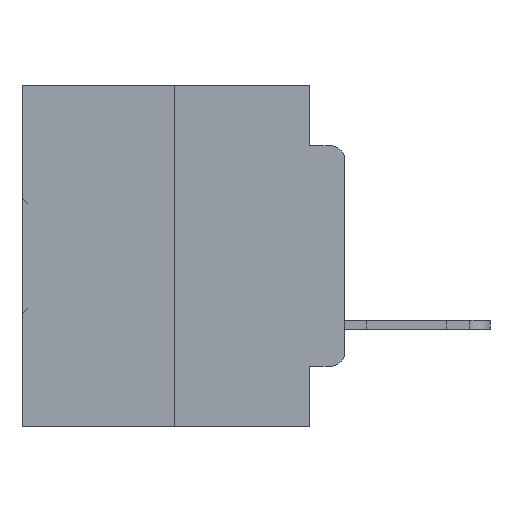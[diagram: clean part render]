
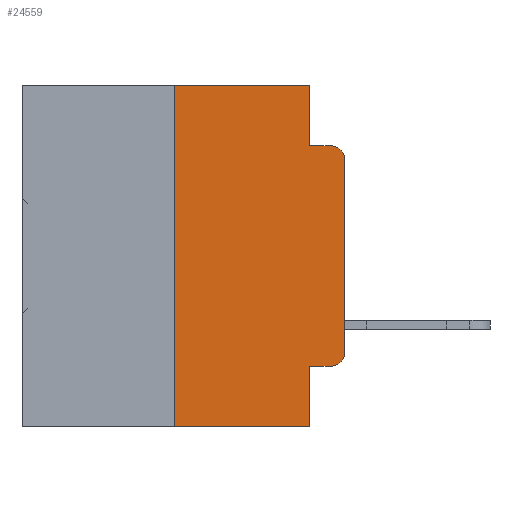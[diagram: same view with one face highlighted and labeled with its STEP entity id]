
A CAD part, left-side view. The second image highlights one B-rep face of the part: STEP entity #24559.
In plain terms, the highlighted planar face has unit normal (-1, 0, 0).
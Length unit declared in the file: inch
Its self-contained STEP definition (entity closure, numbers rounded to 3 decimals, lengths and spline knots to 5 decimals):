
#37 = VECTOR ( 'NONE', #6086, 39.37008 ) ;
#75 = CARTESIAN_POINT ( 'NONE',  ( 0., 0., -0.1085 ) ) ;
#310 = VERTEX_POINT ( 'NONE', #8747 ) ;
#1279 = EDGE_CURVE ( 'NONE', #30486, #15452, #26075, .T. ) ;
#1689 = VECTOR ( 'NONE', #25598, 39.37008 ) ;
#1767 = AXIS2_PLACEMENT_3D ( 'NONE', #25927, #13124, #30879 ) ;
#1870 = CARTESIAN_POINT ( 'NONE',  ( 0., 0.051, 0. ) ) ;
#2720 = LINE ( 'NONE', #21372, #24766 ) ;
#3675 = CARTESIAN_POINT ( 'NONE',  ( 0., 0.051, -0.0885 ) ) ;
#3795 = EDGE_LOOP ( 'NONE', ( #9376, #19537, #5300, #15542, #13757, #17718, #26564, #5742, #23280, #32112 ) ) ;
#3878 = AXIS2_PLACEMENT_3D ( 'NONE', #20931, #21285, #21146 ) ;
#4592 = VECTOR ( 'NONE', #22595, 39.37008 ) ;
#4764 = DIRECTION ( 'NONE',  ( 0., -1., 0. ) ) ;
#4811 = EDGE_CURVE ( 'NONE', #8818, #32693, #23656, .T. ) ;
#5300 = ORIENTED_EDGE ( 'NONE', *, *, #24972, .F. ) ;
#5493 = LINE ( 'NONE', #21628, #31832 ) ;
#5742 = ORIENTED_EDGE ( 'NONE', *, *, #12688, .F. ) ;
#6024 = CARTESIAN_POINT ( 'NONE',  ( 0., 0.051, -0.0885 ) ) ;
#6086 = DIRECTION ( 'NONE',  ( 0., 0., 1. ) ) ;
#6209 = VERTEX_POINT ( 'NONE', #6024 ) ;
#6871 = EDGE_CURVE ( 'NONE', #13027, #8818, #5493, .T. ) ;
#7002 = FACE_OUTER_BOUND ( 'NONE', #3795, .T. ) ;
#7730 = CIRCLE ( 'NONE', #23079, 0.02 ) ;
#8050 = CARTESIAN_POINT ( 'NONE',  ( 0., 0., -0.3915 ) ) ;
#8088 = DIRECTION ( 'NONE',  ( -1., 0., 0. ) ) ;
#8747 = CARTESIAN_POINT ( 'NONE',  ( 0., 0.02, -0.0885 ) ) ;
#8818 = VERTEX_POINT ( 'NONE', #32492 ) ;
#9070 = LINE ( 'NONE', #17429, #23403 ) ;
#9376 = ORIENTED_EDGE ( 'NONE', *, *, #32946, .T. ) ;
#10203 = PLANE ( 'NONE',  #1767 ) ;
#12688 = EDGE_CURVE ( 'NONE', #13027, #26458, #23816, .T. ) ;
#13027 = VERTEX_POINT ( 'NONE', #31003 ) ;
#13124 = DIRECTION ( 'NONE',  ( 1., 0., 0. ) ) ;
#13318 = DIRECTION ( 'NONE',  ( 0., 0., -1. ) ) ;
#13400 = CARTESIAN_POINT ( 'NONE',  ( 0., 0.051, 0. ) ) ;
#13757 = ORIENTED_EDGE ( 'NONE', *, *, #1279, .F. ) ;
#14579 = EDGE_CURVE ( 'NONE', #19467, #30486, #9070, .T. ) ;
#15423 = CARTESIAN_POINT ( 'NONE',  ( 0., 0.25, 0. ) ) ;
#15434 = DIRECTION ( 'NONE',  ( 0., 0., 1. ) ) ;
#15452 = VERTEX_POINT ( 'NONE', #1870 ) ;
#15542 = ORIENTED_EDGE ( 'NONE', *, *, #18186, .F. ) ;
#17429 = CARTESIAN_POINT ( 'NONE',  ( 0., 0.25, 0. ) ) ;
#17718 = ORIENTED_EDGE ( 'NONE', *, *, #14579, .F. ) ;
#17980 = EDGE_CURVE ( 'NONE', #19467, #26458, #2720, .T. ) ;
#18186 = EDGE_CURVE ( 'NONE', #15452, #6209, #25530, .T. ) ;
#19467 = VERTEX_POINT ( 'NONE', #27934 ) ;
#19537 = ORIENTED_EDGE ( 'NONE', *, *, #26612, .T. ) ;
#20770 = DIRECTION ( 'NONE',  ( 0., -1., 0. ) ) ;
#20931 = CARTESIAN_POINT ( 'NONE',  ( 0., 0.02, -0.3915 ) ) ;
#21146 = DIRECTION ( 'NONE',  ( 0., 0., -1. ) ) ;
#21285 = DIRECTION ( 'NONE',  ( -1., 0., 0. ) ) ;
#21372 = CARTESIAN_POINT ( 'NONE',  ( 0., 0.473, -0.5 ) ) ;
#21628 = CARTESIAN_POINT ( 'NONE',  ( 0., 0.051, -0.4115 ) ) ;
#22435 = LINE ( 'NONE', #29793, #37 ) ;
#22595 = DIRECTION ( 'NONE',  ( 0., 0., -1. ) ) ;
#22991 = VECTOR ( 'NONE', #13318, 39.37008 ) ;
#23079 = AXIS2_PLACEMENT_3D ( 'NONE', #24226, #8088, #26688 ) ;
#23280 = ORIENTED_EDGE ( 'NONE', *, *, #6871, .T. ) ;
#23403 = VECTOR ( 'NONE', #15434, 39.37008 ) ;
#23656 = CIRCLE ( 'NONE', #3878, 0.02 ) ;
#23816 = LINE ( 'NONE', #13400, #22991 ) ;
#23888 = LINE ( 'NONE', #3675, #1689 ) ;
#24226 = CARTESIAN_POINT ( 'NONE',  ( 0., 0.02, -0.1085 ) ) ;
#24340 = VERTEX_POINT ( 'NONE', #75 ) ;
#24559 = ADVANCED_FACE ( 'NONE', ( #7002 ), #10203, .F. ) ;
#24766 = VECTOR ( 'NONE', #4764, 39.37008 ) ;
#24972 = EDGE_CURVE ( 'NONE', #6209, #310, #23888, .T. ) ;
#25530 = LINE ( 'NONE', #29918, #4592 ) ;
#25598 = DIRECTION ( 'NONE',  ( 0., -1., 0. ) ) ;
#25927 = CARTESIAN_POINT ( 'NONE',  ( 0., 0.473, 0. ) ) ;
#26075 = LINE ( 'NONE', #27653, #31702 ) ;
#26458 = VERTEX_POINT ( 'NONE', #30465 ) ;
#26564 = ORIENTED_EDGE ( 'NONE', *, *, #17980, .T. ) ;
#26612 = EDGE_CURVE ( 'NONE', #24340, #310, #7730, .T. ) ;
#26688 = DIRECTION ( 'NONE',  ( 0., 0., -1. ) ) ;
#27653 = CARTESIAN_POINT ( 'NONE',  ( 0., 0.473, 0. ) ) ;
#27934 = CARTESIAN_POINT ( 'NONE',  ( 0., 0.25, -0.5 ) ) ;
#29793 = CARTESIAN_POINT ( 'NONE',  ( 0., 0., 0. ) ) ;
#29918 = CARTESIAN_POINT ( 'NONE',  ( 0., 0.051, 0. ) ) ;
#30465 = CARTESIAN_POINT ( 'NONE',  ( 0., 0.051, -0.5 ) ) ;
#30486 = VERTEX_POINT ( 'NONE', #15423 ) ;
#30879 = DIRECTION ( 'NONE',  ( 0., 0., -1. ) ) ;
#31003 = CARTESIAN_POINT ( 'NONE',  ( 0., 0.051, -0.4115 ) ) ;
#31702 = VECTOR ( 'NONE', #33600, 39.37008 ) ;
#31832 = VECTOR ( 'NONE', #20770, 39.37008 ) ;
#32112 = ORIENTED_EDGE ( 'NONE', *, *, #4811, .T. ) ;
#32492 = CARTESIAN_POINT ( 'NONE',  ( 0., 0.02, -0.4115 ) ) ;
#32693 = VERTEX_POINT ( 'NONE', #8050 ) ;
#32946 = EDGE_CURVE ( 'NONE', #32693, #24340, #22435, .T. ) ;
#33600 = DIRECTION ( 'NONE',  ( 0., -1., 0. ) ) ;
